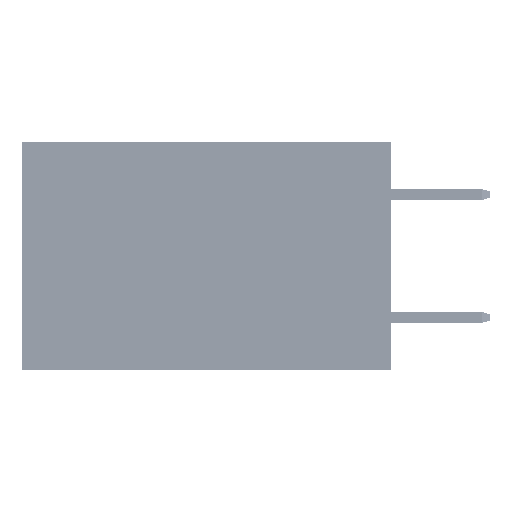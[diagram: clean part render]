
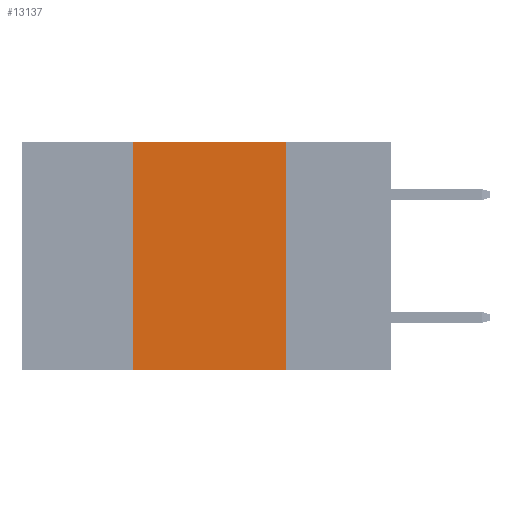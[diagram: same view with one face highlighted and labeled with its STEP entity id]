
A CAD part, left-side view. The second image highlights one B-rep face of the part: STEP entity #13137.
In plain terms, the highlighted planar face has unit normal (-1, 0, 0).
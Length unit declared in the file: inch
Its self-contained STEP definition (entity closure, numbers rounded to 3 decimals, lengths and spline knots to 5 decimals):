
#307 = EDGE_CURVE ( 'NONE', #15852, #8833, #31346, .T. ) ;
#2010 = DIRECTION ( 'NONE',  ( 0., 0., 1. ) ) ;
#5003 = LINE ( 'NONE', #24076, #39079 ) ;
#5943 = EDGE_CURVE ( 'NONE', #47276, #35313, #33636, .T. ) ;
#8833 = VERTEX_POINT ( 'NONE', #9380 ) ;
#9342 = DIRECTION ( 'NONE',  ( 0., 0., -1. ) ) ;
#9380 = CARTESIAN_POINT ( 'NONE',  ( 0., 0.42, 0. ) ) ;
#10046 = FACE_OUTER_BOUND ( 'NONE', #35328, .T. ) ;
#12817 = ORIENTED_EDGE ( 'NONE', *, *, #16345, .F. ) ;
#13137 = ADVANCED_FACE ( 'NONE', ( #10046 ), #17606, .F. ) ;
#13272 = ORIENTED_EDGE ( 'NONE', *, *, #35679, .T. ) ;
#13773 = CARTESIAN_POINT ( 'NONE',  ( 0., 0.6, 0. ) ) ;
#13854 = CARTESIAN_POINT ( 'NONE',  ( 0., 0.42, 0. ) ) ;
#14452 = AXIS2_PLACEMENT_3D ( 'NONE', #13773, #29124, #36465 ) ;
#15112 = DIRECTION ( 'NONE',  ( 0., -1., 0. ) ) ;
#15852 = VERTEX_POINT ( 'NONE', #28325 ) ;
#16345 = EDGE_CURVE ( 'NONE', #8833, #47276, #5003, .T. ) ;
#17606 = PLANE ( 'NONE',  #14452 ) ;
#17621 = CARTESIAN_POINT ( 'NONE',  ( 0., 0.17, -0.37 ) ) ;
#19880 = LINE ( 'NONE', #30271, #28865 ) ;
#20507 = VECTOR ( 'NONE', #9342, 39.37008 ) ;
#21689 = CARTESIAN_POINT ( 'NONE',  ( 0., 0.17, 0. ) ) ;
#23563 = VECTOR ( 'NONE', #2010, 39.37008 ) ;
#24076 = CARTESIAN_POINT ( 'NONE',  ( 0., 0.6, 0. ) ) ;
#28325 = CARTESIAN_POINT ( 'NONE',  ( 0., 0.42, -0.37 ) ) ;
#28551 = ORIENTED_EDGE ( 'NONE', *, *, #307, .F. ) ;
#28865 = VECTOR ( 'NONE', #15112, 39.37008 ) ;
#29124 = DIRECTION ( 'NONE',  ( 1., 0., 0. ) ) ;
#30271 = CARTESIAN_POINT ( 'NONE',  ( 0., 0.6, -0.37 ) ) ;
#31346 = LINE ( 'NONE', #13854, #23563 ) ;
#33560 = ORIENTED_EDGE ( 'NONE', *, *, #5943, .F. ) ;
#33636 = LINE ( 'NONE', #21689, #20507 ) ;
#35313 = VERTEX_POINT ( 'NONE', #17621 ) ;
#35328 = EDGE_LOOP ( 'NONE', ( #33560, #12817, #28551, #13272 ) ) ;
#35679 = EDGE_CURVE ( 'NONE', #15852, #35313, #19880, .T. ) ;
#36465 = DIRECTION ( 'NONE',  ( 0., 0., -1. ) ) ;
#39079 = VECTOR ( 'NONE', #39438, 39.37008 ) ;
#39438 = DIRECTION ( 'NONE',  ( 0., -1., 0. ) ) ;
#41447 = CARTESIAN_POINT ( 'NONE',  ( 0., 0.17, 0. ) ) ;
#47276 = VERTEX_POINT ( 'NONE', #41447 ) ;
